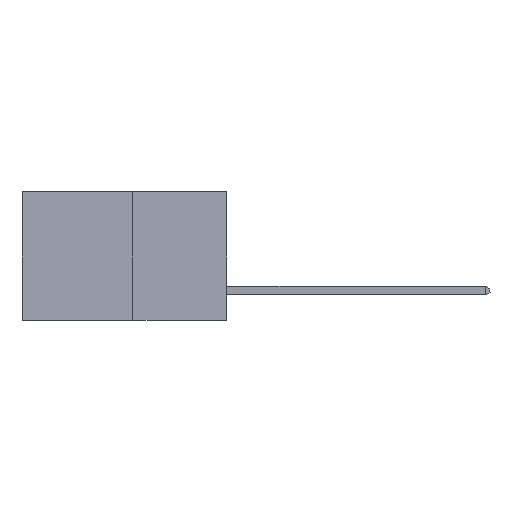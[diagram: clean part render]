
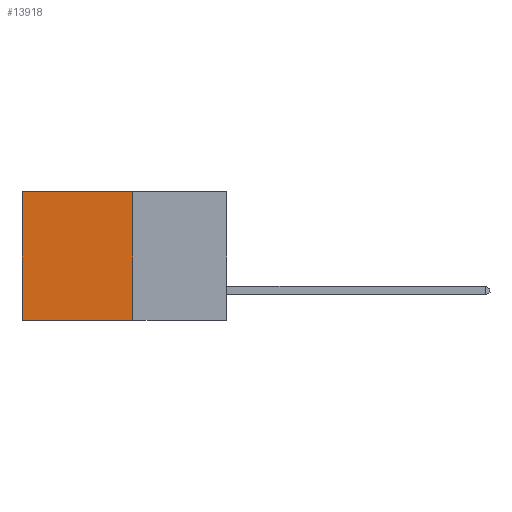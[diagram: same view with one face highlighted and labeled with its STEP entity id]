
A CAD part, left-side view. The second image highlights one B-rep face of the part: STEP entity #13918.
In plain terms, the highlighted planar face has unit normal (-1, 0, 0).
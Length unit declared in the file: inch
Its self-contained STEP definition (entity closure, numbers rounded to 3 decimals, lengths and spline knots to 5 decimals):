
#302 = CARTESIAN_POINT ( 'NONE',  ( 0.277, 0.27, -0.37 ) ) ;
#374 = VECTOR ( 'NONE', #1989, 39.37008 ) ;
#541 = LINE ( 'NONE', #4243, #4298 ) ;
#1003 = EDGE_LOOP ( 'NONE', ( #14761, #11825, #15162, #15569 ) ) ;
#1598 = LINE ( 'NONE', #3098, #7950 ) ;
#1649 = CARTESIAN_POINT ( 'NONE',  ( 0.277, 0.27, -0.37 ) ) ;
#1925 = CARTESIAN_POINT ( 'NONE',  ( 0.277, 0.27, 0. ) ) ;
#1989 = DIRECTION ( 'NONE',  ( 0., 0., -1. ) ) ;
#3060 = CARTESIAN_POINT ( 'NONE',  ( 0.277, 0.59, -0.37 ) ) ;
#3098 = CARTESIAN_POINT ( 'NONE',  ( 0.277, 0.27, -0.37 ) ) ;
#3921 = DIRECTION ( 'NONE',  ( 0., 0., -1. ) ) ;
#4107 = DIRECTION ( 'NONE',  ( 0., 0., -1. ) ) ;
#4181 = VERTEX_POINT ( 'NONE', #1925 ) ;
#4243 = CARTESIAN_POINT ( 'NONE',  ( 0.277, 0.59, -0.37 ) ) ;
#4298 = VECTOR ( 'NONE', #3921, 39.37008 ) ;
#4380 = DIRECTION ( 'NONE',  ( 0., 1., 0. ) ) ;
#5099 = VERTEX_POINT ( 'NONE', #8216 ) ;
#5869 = DIRECTION ( 'NONE',  ( 0., 1., 0. ) ) ;
#6660 = PLANE ( 'NONE',  #7004 ) ;
#6735 = CARTESIAN_POINT ( 'NONE',  ( 0.277, 0.27, 0. ) ) ;
#6986 = VERTEX_POINT ( 'NONE', #3060 ) ;
#7004 = AXIS2_PLACEMENT_3D ( 'NONE', #302, #11656, #4107 ) ;
#7066 = EDGE_CURVE ( 'NONE', #4181, #5099, #13800, .T. ) ;
#7950 = VECTOR ( 'NONE', #4380, 39.37008 ) ;
#7986 = EDGE_CURVE ( 'NONE', #4181, #9344, #10032, .T. ) ;
#8136 = EDGE_CURVE ( 'NONE', #9344, #6986, #541, .T. ) ;
#8216 = CARTESIAN_POINT ( 'NONE',  ( 0.277, 0.27, -0.37 ) ) ;
#9344 = VERTEX_POINT ( 'NONE', #10223 ) ;
#10032 = LINE ( 'NONE', #6735, #15922 ) ;
#10223 = CARTESIAN_POINT ( 'NONE',  ( 0.277, 0.59, 0. ) ) ;
#11656 = DIRECTION ( 'NONE',  ( 1., 0., 0. ) ) ;
#11825 = ORIENTED_EDGE ( 'NONE', *, *, #12753, .F. ) ;
#11894 = FACE_OUTER_BOUND ( 'NONE', #1003, .T. ) ;
#12753 = EDGE_CURVE ( 'NONE', #5099, #6986, #1598, .T. ) ;
#13800 = LINE ( 'NONE', #1649, #374 ) ;
#13918 = ADVANCED_FACE ( 'NONE', ( #11894 ), #6660, .F. ) ;
#14761 = ORIENTED_EDGE ( 'NONE', *, *, #8136, .T. ) ;
#15162 = ORIENTED_EDGE ( 'NONE', *, *, #7066, .F. ) ;
#15569 = ORIENTED_EDGE ( 'NONE', *, *, #7986, .T. ) ;
#15922 = VECTOR ( 'NONE', #5869, 39.37008 ) ;
